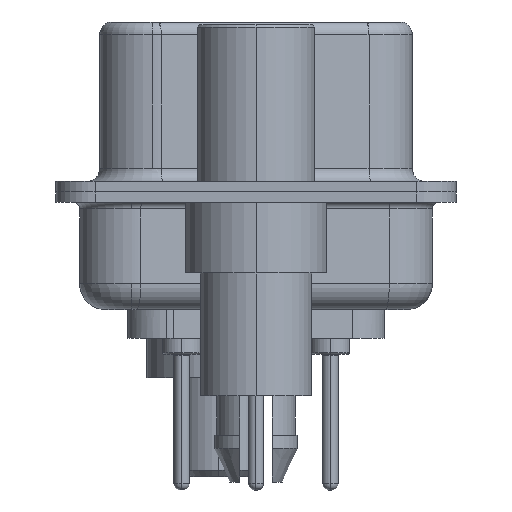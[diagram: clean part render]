
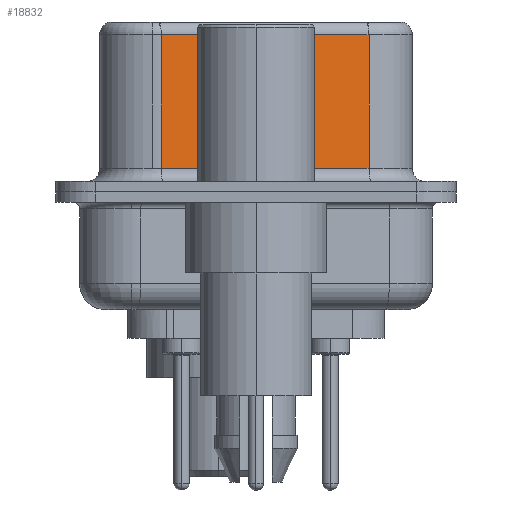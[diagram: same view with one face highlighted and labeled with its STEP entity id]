
A CAD part, left-side view. The second image highlights one B-rep face of the part: STEP entity #18832.
In plain terms, the highlighted planar face has unit normal (-0.985, -0.174, 0).
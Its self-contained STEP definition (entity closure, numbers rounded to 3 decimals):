
#38 = CARTESIAN_POINT ( 'NONE',  ( 5.132, -4.322, 6.02 ) ) ;
#237 = VERTEX_POINT ( 'NONE', #6785 ) ;
#758 = LINE ( 'NONE', #22001, #5796 ) ;
#1833 = ORIENTED_EDGE ( 'NONE', *, *, #5562, .T. ) ;
#2517 = ORIENTED_EDGE ( 'NONE', *, *, #10021, .F. ) ;
#3104 = DIRECTION ( 'NONE',  ( 0., 0., -1. ) ) ;
#4012 = FACE_OUTER_BOUND ( 'NONE', #14138, .T. ) ;
#4478 = CARTESIAN_POINT ( 'NONE',  ( 3.73, 3.628, 0.9 ) ) ;
#5103 = DIRECTION ( 'NONE',  ( 0.174, -0.985, 0. ) ) ;
#5562 = EDGE_CURVE ( 'NONE', #23165, #16181, #14814, .T. ) ;
#5785 = EDGE_CURVE ( 'NONE', #237, #23165, #16644, .T. ) ;
#5796 = VECTOR ( 'NONE', #8176, 1000. ) ;
#5825 = DIRECTION ( 'NONE',  ( 0., 0., -1. ) ) ;
#6785 = CARTESIAN_POINT ( 'NONE',  ( 3.73, 3.628, 6.02 ) ) ;
#7018 = VERTEX_POINT ( 'NONE', #38 ) ;
#7826 = PLANE ( 'NONE',  #19379 ) ;
#8044 = VECTOR ( 'NONE', #5103, 1000. ) ;
#8176 = DIRECTION ( 'NONE',  ( -0.174, 0.985, 0. ) ) ;
#9929 = ORIENTED_EDGE ( 'NONE', *, *, #16216, .T. ) ;
#10021 = EDGE_CURVE ( 'NONE', #7018, #16181, #21503, .T. ) ;
#10530 = VECTOR ( 'NONE', #5825, 1000. ) ;
#10646 = VECTOR ( 'NONE', #3104, 1000. ) ;
#14138 = EDGE_LOOP ( 'NONE', ( #2517, #9929, #29680, #1833 ) ) ;
#14814 = LINE ( 'NONE', #18631, #8044 ) ;
#16181 = VERTEX_POINT ( 'NONE', #28969 ) ;
#16216 = EDGE_CURVE ( 'NONE', #7018, #237, #758, .T. ) ;
#16644 = LINE ( 'NONE', #19652, #10530 ) ;
#17357 = CARTESIAN_POINT ( 'NONE',  ( 5.132, -4.322, 6.52 ) ) ;
#18631 = CARTESIAN_POINT ( 'NONE',  ( 5.132, -4.322, 0.9 ) ) ;
#18832 = ADVANCED_FACE ( 'NONE', ( #4012 ), #7826, .F. ) ;
#19104 = CARTESIAN_POINT ( 'NONE',  ( 5.132, -4.322, 6.52 ) ) ;
#19379 = AXIS2_PLACEMENT_3D ( 'NONE', #17357, #23976, #21847 ) ;
#19652 = CARTESIAN_POINT ( 'NONE',  ( 3.73, 3.628, 6.52 ) ) ;
#21503 = LINE ( 'NONE', #19104, #10646 ) ;
#21847 = DIRECTION ( 'NONE',  ( -0.174, 0.985, 0. ) ) ;
#22001 = CARTESIAN_POINT ( 'NONE',  ( 5.132, -4.322, 6.02 ) ) ;
#23165 = VERTEX_POINT ( 'NONE', #4478 ) ;
#23976 = DIRECTION ( 'NONE',  ( 0.985, 0.174, 0. ) ) ;
#28969 = CARTESIAN_POINT ( 'NONE',  ( 5.132, -4.322, 0.9 ) ) ;
#29680 = ORIENTED_EDGE ( 'NONE', *, *, #5785, .T. ) ;
